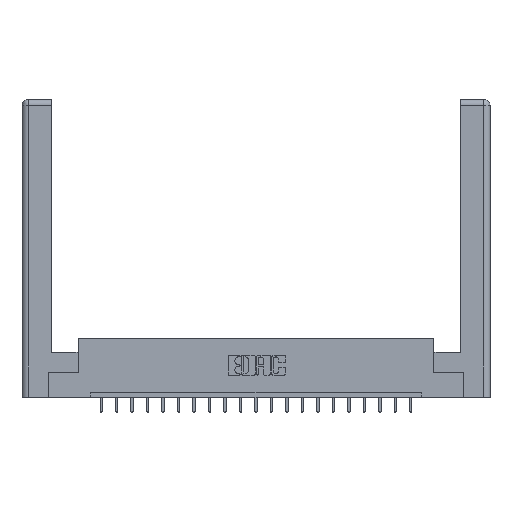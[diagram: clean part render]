
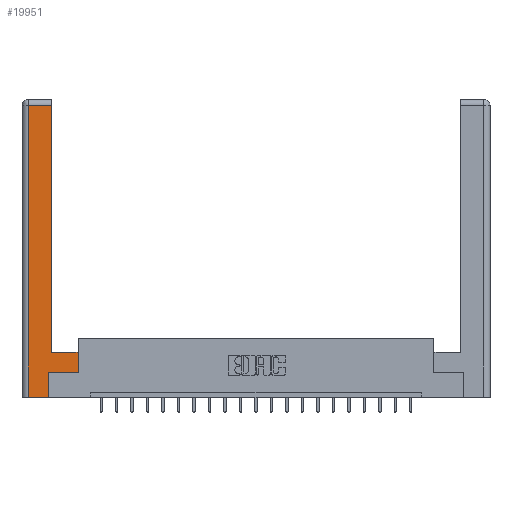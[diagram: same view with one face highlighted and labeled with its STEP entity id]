
A CAD part, top view. The second image highlights one B-rep face of the part: STEP entity #19951.
In plain terms, the highlighted planar face has unit normal (0, 0, 1).
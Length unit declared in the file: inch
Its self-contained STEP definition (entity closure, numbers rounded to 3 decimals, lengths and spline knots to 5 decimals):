
#412 = DIRECTION ( 'NONE',  ( 0., 1., 0. ) ) ;
#428 = VECTOR ( 'NONE', #20501, 39.37008 ) ;
#688 = CARTESIAN_POINT ( 'NONE',  ( 0.265, 0., 0. ) ) ;
#880 = ORIENTED_EDGE ( 'NONE', *, *, #12939, .T. ) ;
#1039 = DIRECTION ( 'NONE',  ( -1., 0., 0. ) ) ;
#1123 = VECTOR ( 'NONE', #12291, 39.37008 ) ;
#1492 = VECTOR ( 'NONE', #412, 39.37008 ) ;
#1731 = LINE ( 'NONE', #6795, #1492 ) ;
#2369 = VECTOR ( 'NONE', #14327, 39.37008 ) ;
#2525 = VECTOR ( 'NONE', #14947, 39.37008 ) ;
#3668 = CARTESIAN_POINT ( 'NONE',  ( 0.565, 0.45, 0. ) ) ;
#3877 = PLANE ( 'NONE',  #17069 ) ;
#4156 = FACE_OUTER_BOUND ( 'NONE', #20965, .T. ) ;
#4451 = CARTESIAN_POINT ( 'NONE',  ( 0.565, 0.45, 0. ) ) ;
#4632 = LINE ( 'NONE', #12906, #9417 ) ;
#5144 = EDGE_CURVE ( 'NONE', #9676, #20200, #4632, .T. ) ;
#5354 = LINE ( 'NONE', #13628, #12962 ) ;
#5816 = ORIENTED_EDGE ( 'NONE', *, *, #12791, .T. ) ;
#6077 = CARTESIAN_POINT ( 'NONE',  ( 0., 0., 0. ) ) ;
#6795 = CARTESIAN_POINT ( 'NONE',  ( 0.265, 0.245, 0. ) ) ;
#7729 = LINE ( 'NONE', #20324, #1123 ) ;
#7819 = ORIENTED_EDGE ( 'NONE', *, *, #18667, .T. ) ;
#8362 = CARTESIAN_POINT ( 'NONE',  ( 0.0615, 0., 0. ) ) ;
#8517 = CARTESIAN_POINT ( 'NONE',  ( 0.0615, 2.94, 0. ) ) ;
#8583 = ORIENTED_EDGE ( 'NONE', *, *, #14756, .T. ) ;
#9417 = VECTOR ( 'NONE', #12974, 39.37008 ) ;
#9676 = VERTEX_POINT ( 'NONE', #19246 ) ;
#10922 = VERTEX_POINT ( 'NONE', #11084 ) ;
#11084 = CARTESIAN_POINT ( 'NONE',  ( 0.0615, 0., 0. ) ) ;
#11155 = VERTEX_POINT ( 'NONE', #18184 ) ;
#11701 = DIRECTION ( 'NONE',  ( -1., 0., 0. ) ) ;
#11803 = LINE ( 'NONE', #20879, #2369 ) ;
#11879 = VERTEX_POINT ( 'NONE', #18622 ) ;
#12041 = DIRECTION ( 'NONE',  ( 1., 0., 0. ) ) ;
#12291 = DIRECTION ( 'NONE',  ( -1., 0., 0. ) ) ;
#12440 = EDGE_CURVE ( 'NONE', #18619, #9676, #5354, .T. ) ;
#12791 = EDGE_CURVE ( 'NONE', #16910, #10922, #16000, .T. ) ;
#12897 = ORIENTED_EDGE ( 'NONE', *, *, #19563, .T. ) ;
#12906 = CARTESIAN_POINT ( 'NONE',  ( 0.295, 3., 0. ) ) ;
#12939 = EDGE_CURVE ( 'NONE', #10922, #11879, #16981, .T. ) ;
#12962 = VECTOR ( 'NONE', #11701, 39.37008 ) ;
#12974 = DIRECTION ( 'NONE',  ( 0., 1., 0. ) ) ;
#13022 = ORIENTED_EDGE ( 'NONE', *, *, #12440, .T. ) ;
#13628 = CARTESIAN_POINT ( 'NONE',  ( 0.295, 0.45, 0. ) ) ;
#14327 = DIRECTION ( 'NONE',  ( 1., 0., 0. ) ) ;
#14756 = EDGE_CURVE ( 'NONE', #11155, #18619, #17888, .T. ) ;
#14853 = ORIENTED_EDGE ( 'NONE', *, *, #5144, .T. ) ;
#14947 = DIRECTION ( 'NONE',  ( 0., -1., 0. ) ) ;
#15723 = DIRECTION ( 'NONE',  ( 0., 0., -1. ) ) ;
#16000 = LINE ( 'NONE', #8362, #2525 ) ;
#16219 = EDGE_CURVE ( 'NONE', #11879, #16345, #1731, .T. ) ;
#16345 = VERTEX_POINT ( 'NONE', #17473 ) ;
#16801 = CARTESIAN_POINT ( 'NONE',  ( 0.295, 2.94, 0. ) ) ;
#16910 = VERTEX_POINT ( 'NONE', #8517 ) ;
#16981 = LINE ( 'NONE', #688, #17482 ) ;
#17069 = AXIS2_PLACEMENT_3D ( 'NONE', #6077, #15723, #1039 ) ;
#17473 = CARTESIAN_POINT ( 'NONE',  ( 0.265, 0.245, 0. ) ) ;
#17482 = VECTOR ( 'NONE', #12041, 39.37008 ) ;
#17888 = LINE ( 'NONE', #4451, #428 ) ;
#18184 = CARTESIAN_POINT ( 'NONE',  ( 0.565, 0.245, 0. ) ) ;
#18619 = VERTEX_POINT ( 'NONE', #3668 ) ;
#18622 = CARTESIAN_POINT ( 'NONE',  ( 0.265, 0., 0. ) ) ;
#18667 = EDGE_CURVE ( 'NONE', #16345, #11155, #11803, .T. ) ;
#18875 = ORIENTED_EDGE ( 'NONE', *, *, #16219, .T. ) ;
#19246 = CARTESIAN_POINT ( 'NONE',  ( 0.295, 0.45, 0. ) ) ;
#19563 = EDGE_CURVE ( 'NONE', #20200, #16910, #7729, .T. ) ;
#19951 = ADVANCED_FACE ( 'NONE', ( #4156 ), #3877, .F. ) ;
#20200 = VERTEX_POINT ( 'NONE', #16801 ) ;
#20324 = CARTESIAN_POINT ( 'NONE',  ( 0.0615, 2.94, 0. ) ) ;
#20501 = DIRECTION ( 'NONE',  ( 0., 1., 0. ) ) ;
#20879 = CARTESIAN_POINT ( 'NONE',  ( 0.565, 0.245, 0. ) ) ;
#20965 = EDGE_LOOP ( 'NONE', ( #14853, #12897, #5816, #880, #18875, #7819, #8583, #13022 ) ) ;
